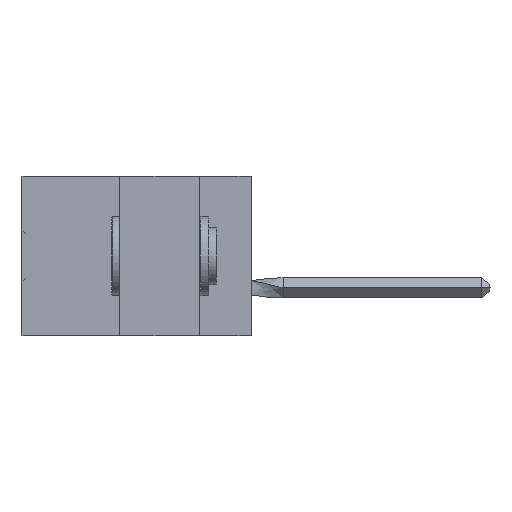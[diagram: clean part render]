
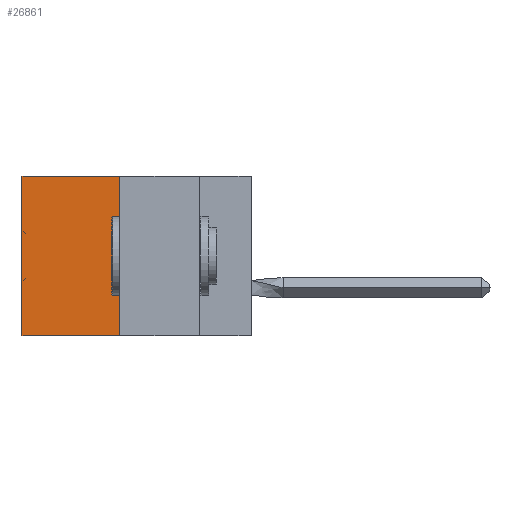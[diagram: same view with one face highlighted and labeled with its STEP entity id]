
A CAD part, left-side view. The second image highlights one B-rep face of the part: STEP entity #26861.
In plain terms, the highlighted planar face has unit normal (-1, 0, 0).
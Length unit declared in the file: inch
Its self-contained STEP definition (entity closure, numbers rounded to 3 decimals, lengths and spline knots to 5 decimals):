
#980 = ORIENTED_EDGE ( 'NONE', *, *, #28429, .F. ) ;
#3544 = VECTOR ( 'NONE', #48202, 39.37008 ) ;
#9055 = EDGE_CURVE ( 'NONE', #17753, #41838, #27724, .T. ) ;
#9227 = VERTEX_POINT ( 'NONE', #32242 ) ;
#11564 = AXIS2_PLACEMENT_3D ( 'NONE', #42647, #51208, #37957 ) ;
#15345 = EDGE_LOOP ( 'NONE', ( #19333, #52111, #980, #38622 ) ) ;
#17753 = VERTEX_POINT ( 'NONE', #44069 ) ;
#19333 = ORIENTED_EDGE ( 'NONE', *, *, #35182, .T. ) ;
#19724 = PLANE ( 'NONE',  #11564 ) ;
#20403 = DIRECTION ( 'NONE',  ( 0., 0., -1. ) ) ;
#21087 = DIRECTION ( 'NONE',  ( 0., 1., 0. ) ) ;
#22969 = CARTESIAN_POINT ( 'NONE',  ( 0.305, 0.413, -0.5 ) ) ;
#23413 = EDGE_CURVE ( 'NONE', #40238, #9227, #50966, .T. ) ;
#26861 = ADVANCED_FACE ( 'NONE', ( #52070 ), #19724, .F. ) ;
#27724 = LINE ( 'NONE', #47709, #43016 ) ;
#28002 = CARTESIAN_POINT ( 'NONE',  ( 0.305, 0.413, -0.5 ) ) ;
#28429 = EDGE_CURVE ( 'NONE', #17753, #40238, #53175, .T. ) ;
#29194 = CARTESIAN_POINT ( 'NONE',  ( 0.305, 0.72, -0.5 ) ) ;
#32242 = CARTESIAN_POINT ( 'NONE',  ( 0.305, 0.72, -0.5 ) ) ;
#35067 = VECTOR ( 'NONE', #20403, 39.37008 ) ;
#35182 = EDGE_CURVE ( 'NONE', #41838, #9227, #40403, .T. ) ;
#37957 = DIRECTION ( 'NONE',  ( 0., 0., -1. ) ) ;
#38622 = ORIENTED_EDGE ( 'NONE', *, *, #9055, .T. ) ;
#40238 = VERTEX_POINT ( 'NONE', #49649 ) ;
#40403 = LINE ( 'NONE', #29194, #3544 ) ;
#41243 = DIRECTION ( 'NONE',  ( 0., 1., 0. ) ) ;
#41838 = VERTEX_POINT ( 'NONE', #54070 ) ;
#42647 = CARTESIAN_POINT ( 'NONE',  ( 0.305, 0.413, -0.5 ) ) ;
#43016 = VECTOR ( 'NONE', #21087, 39.37008 ) ;
#44069 = CARTESIAN_POINT ( 'NONE',  ( 0.305, 0.413, 0. ) ) ;
#47709 = CARTESIAN_POINT ( 'NONE',  ( 0.305, 0.413, 0. ) ) ;
#48116 = VECTOR ( 'NONE', #41243, 39.37008 ) ;
#48202 = DIRECTION ( 'NONE',  ( 0., 0., -1. ) ) ;
#49649 = CARTESIAN_POINT ( 'NONE',  ( 0.305, 0.413, -0.5 ) ) ;
#50966 = LINE ( 'NONE', #22969, #48116 ) ;
#51208 = DIRECTION ( 'NONE',  ( 1., 0., 0. ) ) ;
#52070 = FACE_OUTER_BOUND ( 'NONE', #15345, .T. ) ;
#52111 = ORIENTED_EDGE ( 'NONE', *, *, #23413, .F. ) ;
#53175 = LINE ( 'NONE', #28002, #35067 ) ;
#54070 = CARTESIAN_POINT ( 'NONE',  ( 0.305, 0.72, 0. ) ) ;
